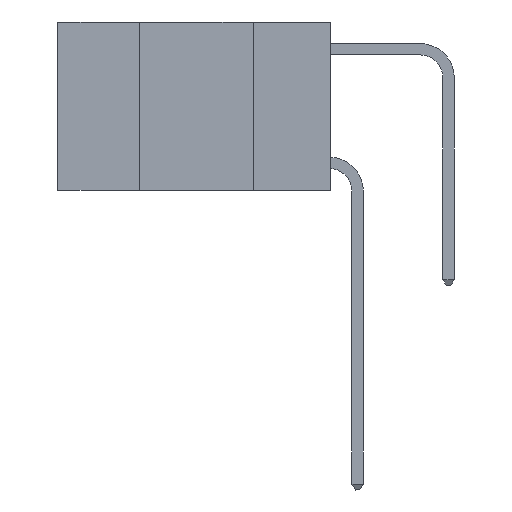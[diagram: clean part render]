
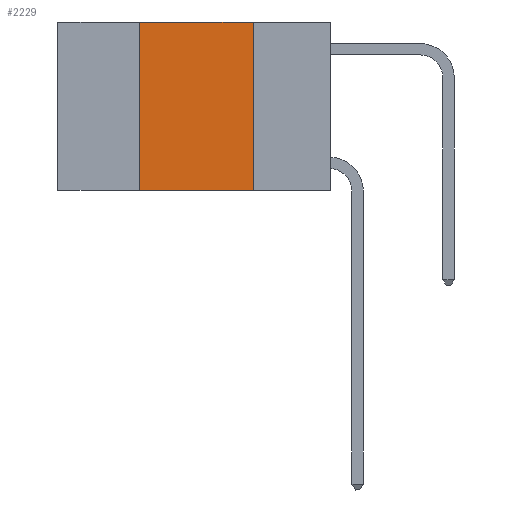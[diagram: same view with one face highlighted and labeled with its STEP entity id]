
A CAD part, left-side view. The second image highlights one B-rep face of the part: STEP entity #2229.
In plain terms, the highlighted planar face has unit normal (-1, 0, 0).
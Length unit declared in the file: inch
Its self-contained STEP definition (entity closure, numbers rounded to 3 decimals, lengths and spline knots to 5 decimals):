
#3 = EDGE_CURVE ( 'NONE', #7183, #8804, #3422, .T. ) ;
#84 = EDGE_CURVE ( 'NONE', #7183, #1167, #11044, .T. ) ;
#104 = AXIS2_PLACEMENT_3D ( 'NONE', #4443, #9622, #9328 ) ;
#193 = EDGE_CURVE ( 'NONE', #10930, #1167, #930, .T. ) ;
#537 = DIRECTION ( 'NONE',  ( 0., -1., 0. ) ) ;
#600 = VECTOR ( 'NONE', #1091, 39.37008 ) ;
#930 = LINE ( 'NONE', #2656, #1268 ) ;
#1091 = DIRECTION ( 'NONE',  ( 0., 0., 1. ) ) ;
#1167 = VERTEX_POINT ( 'NONE', #1468 ) ;
#1268 = VECTOR ( 'NONE', #4265, 39.37008 ) ;
#1468 = CARTESIAN_POINT ( 'NONE',  ( 0., 0.17, -0.37 ) ) ;
#1778 = VECTOR ( 'NONE', #537, 39.37008 ) ;
#1809 = CARTESIAN_POINT ( 'NONE',  ( 0., 0.42, 0. ) ) ;
#2150 = CARTESIAN_POINT ( 'NONE',  ( 0., 0.42, 0. ) ) ;
#2229 = ADVANCED_FACE ( 'NONE', ( #8679 ), #4350, .F. ) ;
#2566 = DIRECTION ( 'NONE',  ( 0., -1., 0. ) ) ;
#2656 = CARTESIAN_POINT ( 'NONE',  ( 0., 0.17, 0. ) ) ;
#3422 = LINE ( 'NONE', #1809, #600 ) ;
#4052 = EDGE_CURVE ( 'NONE', #8804, #10930, #4807, .T. ) ;
#4265 = DIRECTION ( 'NONE',  ( 0., 0., -1. ) ) ;
#4350 = PLANE ( 'NONE',  #104 ) ;
#4443 = CARTESIAN_POINT ( 'NONE',  ( 0., 0.6, 0. ) ) ;
#4807 = LINE ( 'NONE', #9543, #6904 ) ;
#4942 = ORIENTED_EDGE ( 'NONE', *, *, #84, .T. ) ;
#4992 = ORIENTED_EDGE ( 'NONE', *, *, #3, .F. ) ;
#5083 = ORIENTED_EDGE ( 'NONE', *, *, #4052, .F. ) ;
#5113 = ORIENTED_EDGE ( 'NONE', *, *, #193, .F. ) ;
#6348 = EDGE_LOOP ( 'NONE', ( #5113, #5083, #4992, #4942 ) ) ;
#6634 = CARTESIAN_POINT ( 'NONE',  ( 0., 0.42, -0.37 ) ) ;
#6904 = VECTOR ( 'NONE', #2566, 39.37008 ) ;
#7183 = VERTEX_POINT ( 'NONE', #6634 ) ;
#8679 = FACE_OUTER_BOUND ( 'NONE', #6348, .T. ) ;
#8804 = VERTEX_POINT ( 'NONE', #2150 ) ;
#9328 = DIRECTION ( 'NONE',  ( 0., 0., -1. ) ) ;
#9543 = CARTESIAN_POINT ( 'NONE',  ( 0., 0.6, 0. ) ) ;
#9622 = DIRECTION ( 'NONE',  ( 1., 0., 0. ) ) ;
#10509 = CARTESIAN_POINT ( 'NONE',  ( 0., 0.6, -0.37 ) ) ;
#10930 = VERTEX_POINT ( 'NONE', #11439 ) ;
#11044 = LINE ( 'NONE', #10509, #1778 ) ;
#11439 = CARTESIAN_POINT ( 'NONE',  ( 0., 0.17, 0. ) ) ;
